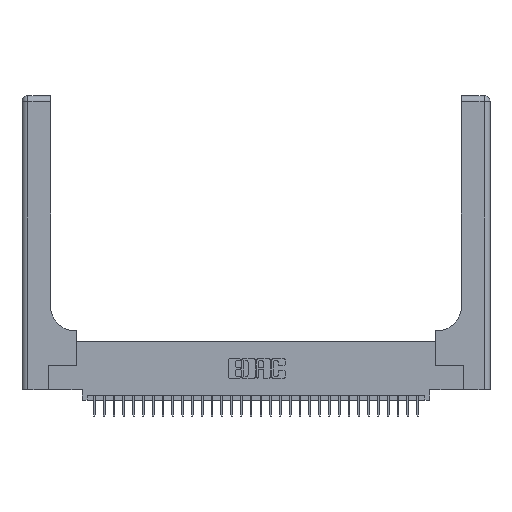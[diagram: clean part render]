
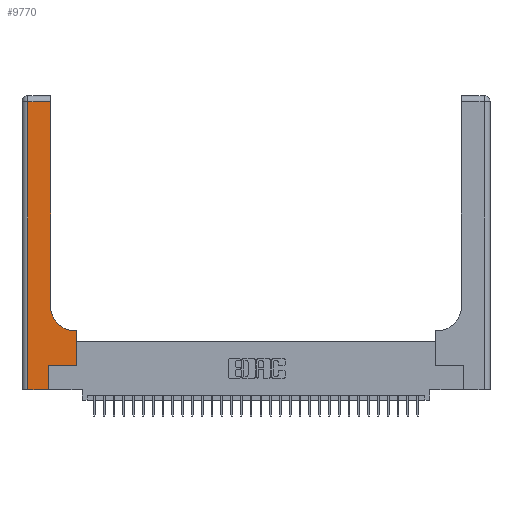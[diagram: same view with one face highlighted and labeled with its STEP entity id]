
A CAD part, top view. The second image highlights one B-rep face of the part: STEP entity #9770.
In plain terms, the highlighted planar face has unit normal (0, 0, 1).
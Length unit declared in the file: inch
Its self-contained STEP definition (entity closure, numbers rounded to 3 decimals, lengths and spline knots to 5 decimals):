
#689 = CIRCLE ( 'NONE', #13660, 0.25 ) ;
#966 = EDGE_LOOP ( 'NONE', ( #30946, #14408, #20662, #8288, #26301, #1032, #14842, #16786, #19376 ) ) ;
#1032 = ORIENTED_EDGE ( 'NONE', *, *, #8029, .T. ) ;
#1135 = LINE ( 'NONE', #23088, #17952 ) ;
#1817 = VECTOR ( 'NONE', #12766, 39.37008 ) ;
#2041 = VERTEX_POINT ( 'NONE', #6104 ) ;
#2207 = VECTOR ( 'NONE', #18574, 39.37008 ) ;
#2860 = EDGE_CURVE ( 'NONE', #22025, #22332, #689, .T. ) ;
#2952 = DIRECTION ( 'NONE',  ( 0., -1., 0. ) ) ;
#5309 = VERTEX_POINT ( 'NONE', #24585 ) ;
#6104 = CARTESIAN_POINT ( 'NONE',  ( 0.5585, 0.6, 0.37 ) ) ;
#6527 = EDGE_CURVE ( 'NONE', #21382, #23807, #32916, .T. ) ;
#7046 = EDGE_CURVE ( 'NONE', #23807, #22947, #28432, .T. ) ;
#7667 = DIRECTION ( 'NONE',  ( 0., 1., 0. ) ) ;
#8029 = EDGE_CURVE ( 'NONE', #22947, #31698, #1135, .T. ) ;
#8288 = ORIENTED_EDGE ( 'NONE', *, *, #6527, .T. ) ;
#9264 = DIRECTION ( 'NONE',  ( 0., 0., -1. ) ) ;
#9743 = LINE ( 'NONE', #30294, #18509 ) ;
#9770 = ADVANCED_FACE ( 'NONE', ( #21503 ), #14632, .F. ) ;
#10828 = VECTOR ( 'NONE', #23508, 39.37008 ) ;
#11077 = EDGE_CURVE ( 'NONE', #2041, #22025, #15789, .T. ) ;
#12766 = DIRECTION ( 'NONE',  ( -1., 0., 0. ) ) ;
#13607 = LINE ( 'NONE', #26317, #10828 ) ;
#13660 = AXIS2_PLACEMENT_3D ( 'NONE', #32205, #9264, #21483 ) ;
#14408 = ORIENTED_EDGE ( 'NONE', *, *, #14685, .T. ) ;
#14632 = PLANE ( 'NONE',  #32697 ) ;
#14685 = EDGE_CURVE ( 'NONE', #18587, #5309, #26228, .T. ) ;
#14842 = ORIENTED_EDGE ( 'NONE', *, *, #29865, .T. ) ;
#15789 = LINE ( 'NONE', #28674, #2207 ) ;
#15891 = EDGE_CURVE ( 'NONE', #22332, #18587, #9743, .T. ) ;
#16330 = CARTESIAN_POINT ( 'NONE',  ( 0.2915, 0.85, 0.37 ) ) ;
#16531 = CARTESIAN_POINT ( 'NONE',  ( 0.269, 0., 0.37 ) ) ;
#16786 = ORIENTED_EDGE ( 'NONE', *, *, #11077, .T. ) ;
#17652 = CARTESIAN_POINT ( 'NONE',  ( 0.06, 0., 0.37 ) ) ;
#17952 = VECTOR ( 'NONE', #28142, 39.37008 ) ;
#17964 = EDGE_CURVE ( 'NONE', #5309, #21382, #28392, .T. ) ;
#18509 = VECTOR ( 'NONE', #7667, 39.37008 ) ;
#18574 = DIRECTION ( 'NONE',  ( -1., 0., 0. ) ) ;
#18587 = VERTEX_POINT ( 'NONE', #19278 ) ;
#18943 = CARTESIAN_POINT ( 'NONE',  ( 0., 0., 0.37 ) ) ;
#19278 = CARTESIAN_POINT ( 'NONE',  ( 0.2915, 2.94, 0.37 ) ) ;
#19376 = ORIENTED_EDGE ( 'NONE', *, *, #2860, .T. ) ;
#20662 = ORIENTED_EDGE ( 'NONE', *, *, #17964, .T. ) ;
#20715 = CARTESIAN_POINT ( 'NONE',  ( 0.5415, 0.6, 0.37 ) ) ;
#21382 = VERTEX_POINT ( 'NONE', #17652 ) ;
#21427 = CARTESIAN_POINT ( 'NONE',  ( 0.269, 0., 0.37 ) ) ;
#21483 = DIRECTION ( 'NONE',  ( 1., 0., 0. ) ) ;
#21503 = FACE_OUTER_BOUND ( 'NONE', #966, .T. ) ;
#22025 = VERTEX_POINT ( 'NONE', #20715 ) ;
#22332 = VERTEX_POINT ( 'NONE', #16330 ) ;
#22715 = CARTESIAN_POINT ( 'NONE',  ( 0., 3., 0.37 ) ) ;
#22856 = VECTOR ( 'NONE', #26954, 39.37008 ) ;
#22947 = VERTEX_POINT ( 'NONE', #30461 ) ;
#22967 = CARTESIAN_POINT ( 'NONE',  ( 0., 2.94, 0.37 ) ) ;
#23088 = CARTESIAN_POINT ( 'NONE',  ( 0.269, 0.25, 0.37 ) ) ;
#23508 = DIRECTION ( 'NONE',  ( 0., 1., 0. ) ) ;
#23654 = VECTOR ( 'NONE', #24067, 39.37008 ) ;
#23807 = VERTEX_POINT ( 'NONE', #21427 ) ;
#24067 = DIRECTION ( 'NONE',  ( 1., 0., 0. ) ) ;
#24585 = CARTESIAN_POINT ( 'NONE',  ( 0.06, 2.94, 0.37 ) ) ;
#25394 = DIRECTION ( 'NONE',  ( 0., 0., -1. ) ) ;
#25545 = CARTESIAN_POINT ( 'NONE',  ( 0.5585, 0.25, 0.37 ) ) ;
#25598 = VECTOR ( 'NONE', #2952, 39.37008 ) ;
#26228 = LINE ( 'NONE', #22967, #1817 ) ;
#26301 = ORIENTED_EDGE ( 'NONE', *, *, #7046, .T. ) ;
#26317 = CARTESIAN_POINT ( 'NONE',  ( 0.5585, 0.25, 0.37 ) ) ;
#26954 = DIRECTION ( 'NONE',  ( 0., 1., 0. ) ) ;
#28142 = DIRECTION ( 'NONE',  ( 1., 0., 0. ) ) ;
#28392 = LINE ( 'NONE', #31392, #25598 ) ;
#28432 = LINE ( 'NONE', #16531, #22856 ) ;
#28674 = CARTESIAN_POINT ( 'NONE',  ( 0.2915, 0.6, 0.37 ) ) ;
#29865 = EDGE_CURVE ( 'NONE', #31698, #2041, #13607, .T. ) ;
#30294 = CARTESIAN_POINT ( 'NONE',  ( 0.2915, 3., 0.37 ) ) ;
#30461 = CARTESIAN_POINT ( 'NONE',  ( 0.269, 0.25, 0.37 ) ) ;
#30946 = ORIENTED_EDGE ( 'NONE', *, *, #15891, .T. ) ;
#31392 = CARTESIAN_POINT ( 'NONE',  ( 0.06, 3., 0.37 ) ) ;
#31698 = VERTEX_POINT ( 'NONE', #25545 ) ;
#32205 = CARTESIAN_POINT ( 'NONE',  ( 0.5415, 0.85, 0.37 ) ) ;
#32685 = DIRECTION ( 'NONE',  ( -1., 0., 0. ) ) ;
#32697 = AXIS2_PLACEMENT_3D ( 'NONE', #22715, #25394, #32685 ) ;
#32916 = LINE ( 'NONE', #18943, #23654 ) ;
